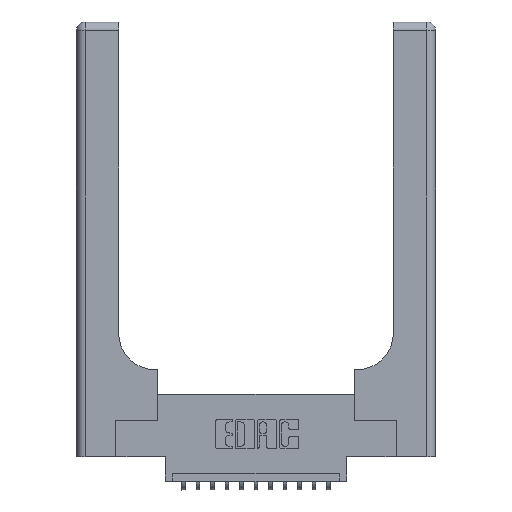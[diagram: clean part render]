
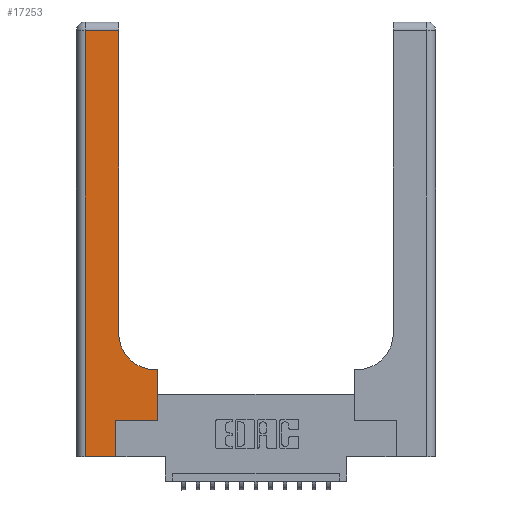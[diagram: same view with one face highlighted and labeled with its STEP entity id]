
A CAD part, top view. The second image highlights one B-rep face of the part: STEP entity #17253.
In plain terms, the highlighted planar face has unit normal (0, 0, 1).
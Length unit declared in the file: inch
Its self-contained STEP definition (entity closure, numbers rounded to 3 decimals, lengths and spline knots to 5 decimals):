
#71 = CARTESIAN_POINT ( 'NONE',  ( 0.269, 0.25, 0.37 ) ) ;
#83 = ORIENTED_EDGE ( 'NONE', *, *, #8795, .T. ) ;
#147 = AXIS2_PLACEMENT_3D ( 'NONE', #15369, #10408, #6244 ) ;
#502 = ORIENTED_EDGE ( 'NONE', *, *, #13716, .T. ) ;
#949 = EDGE_CURVE ( 'NONE', #11735, #5398, #17181, .T. ) ;
#1242 = CARTESIAN_POINT ( 'NONE',  ( 0.06, 3., 0.37 ) ) ;
#1856 = CARTESIAN_POINT ( 'NONE',  ( 0.06, 2.94, 0.37 ) ) ;
#2227 = DIRECTION ( 'NONE',  ( 0., 1., 0. ) ) ;
#2229 = CIRCLE ( 'NONE', #8083, 0.25 ) ;
#2405 = CARTESIAN_POINT ( 'NONE',  ( 0.269, 0., 0.37 ) ) ;
#2759 = VECTOR ( 'NONE', #15936, 39.37008 ) ;
#2775 = CARTESIAN_POINT ( 'NONE',  ( 0.06, 0., 0.37 ) ) ;
#2853 = CARTESIAN_POINT ( 'NONE',  ( 0.5585, 0.6, 0.37 ) ) ;
#2884 = VERTEX_POINT ( 'NONE', #9789 ) ;
#2964 = DIRECTION ( 'NONE',  ( 1., 0., 0. ) ) ;
#3438 = LINE ( 'NONE', #71, #13962 ) ;
#3503 = CARTESIAN_POINT ( 'NONE',  ( 0.2915, 3., 0.37 ) ) ;
#3720 = ORIENTED_EDGE ( 'NONE', *, *, #6353, .T. ) ;
#4133 = DIRECTION ( 'NONE',  ( 0., -1., 0. ) ) ;
#4957 = DIRECTION ( 'NONE',  ( -1., 0., 0. ) ) ;
#4966 = ORIENTED_EDGE ( 'NONE', *, *, #13176, .T. ) ;
#5148 = CARTESIAN_POINT ( 'NONE',  ( 0.5585, 0.25, 0.37 ) ) ;
#5274 = ORIENTED_EDGE ( 'NONE', *, *, #8549, .T. ) ;
#5398 = VERTEX_POINT ( 'NONE', #16535 ) ;
#5420 = VERTEX_POINT ( 'NONE', #6772 ) ;
#5808 = EDGE_LOOP ( 'NONE', ( #17011, #8208, #502, #4966, #7410, #14130, #3720, #83, #5274 ) ) ;
#6244 = DIRECTION ( 'NONE',  ( -1., 0., 0. ) ) ;
#6353 = EDGE_CURVE ( 'NONE', #7748, #11302, #6376, .T. ) ;
#6376 = LINE ( 'NONE', #5148, #11533 ) ;
#6515 = LINE ( 'NONE', #16203, #10816 ) ;
#6772 = CARTESIAN_POINT ( 'NONE',  ( 0.2915, 0.85, 0.37 ) ) ;
#7296 = VECTOR ( 'NONE', #2227, 39.37008 ) ;
#7410 = ORIENTED_EDGE ( 'NONE', *, *, #949, .T. ) ;
#7748 = VERTEX_POINT ( 'NONE', #16644 ) ;
#8083 = AXIS2_PLACEMENT_3D ( 'NONE', #11205, #10980, #2964 ) ;
#8169 = EDGE_CURVE ( 'NONE', #2884, #17229, #13679, .T. ) ;
#8208 = ORIENTED_EDGE ( 'NONE', *, *, #8169, .T. ) ;
#8503 = DIRECTION ( 'NONE',  ( 1., 0., 0. ) ) ;
#8549 = EDGE_CURVE ( 'NONE', #12171, #5420, #2229, .T. ) ;
#8795 = EDGE_CURVE ( 'NONE', #11302, #12171, #13235, .T. ) ;
#9048 = VERTEX_POINT ( 'NONE', #2775 ) ;
#9116 = CARTESIAN_POINT ( 'NONE',  ( 0.269, 0., 0.37 ) ) ;
#9351 = DIRECTION ( 'NONE',  ( -1., 0., 0. ) ) ;
#9527 = VECTOR ( 'NONE', #9351, 39.37008 ) ;
#9565 = VECTOR ( 'NONE', #4957, 39.37008 ) ;
#9789 = CARTESIAN_POINT ( 'NONE',  ( 0.2915, 2.94, 0.37 ) ) ;
#10408 = DIRECTION ( 'NONE',  ( 0., 0., -1. ) ) ;
#10785 = EDGE_CURVE ( 'NONE', #5420, #2884, #12293, .T. ) ;
#10816 = VECTOR ( 'NONE', #12349, 39.37008 ) ;
#10980 = DIRECTION ( 'NONE',  ( 0., 0., -1. ) ) ;
#11205 = CARTESIAN_POINT ( 'NONE',  ( 0.5415, 0.85, 0.37 ) ) ;
#11302 = VERTEX_POINT ( 'NONE', #2853 ) ;
#11391 = CARTESIAN_POINT ( 'NONE',  ( 0.5415, 0.6, 0.37 ) ) ;
#11533 = VECTOR ( 'NONE', #14836, 39.37008 ) ;
#11735 = VERTEX_POINT ( 'NONE', #9116 ) ;
#12171 = VERTEX_POINT ( 'NONE', #11391 ) ;
#12293 = LINE ( 'NONE', #3503, #7296 ) ;
#12315 = VECTOR ( 'NONE', #4133, 39.37008 ) ;
#12349 = DIRECTION ( 'NONE',  ( 1., 0., 0. ) ) ;
#12642 = PLANE ( 'NONE',  #147 ) ;
#13176 = EDGE_CURVE ( 'NONE', #9048, #11735, #6515, .T. ) ;
#13198 = LINE ( 'NONE', #1242, #12315 ) ;
#13232 = CARTESIAN_POINT ( 'NONE',  ( 0., 2.94, 0.37 ) ) ;
#13235 = LINE ( 'NONE', #16403, #9527 ) ;
#13679 = LINE ( 'NONE', #13232, #9565 ) ;
#13716 = EDGE_CURVE ( 'NONE', #17229, #9048, #13198, .T. ) ;
#13962 = VECTOR ( 'NONE', #8503, 39.37008 ) ;
#14130 = ORIENTED_EDGE ( 'NONE', *, *, #15879, .T. ) ;
#14563 = FACE_OUTER_BOUND ( 'NONE', #5808, .T. ) ;
#14836 = DIRECTION ( 'NONE',  ( 0., 1., 0. ) ) ;
#15369 = CARTESIAN_POINT ( 'NONE',  ( 0., 3., 0.37 ) ) ;
#15879 = EDGE_CURVE ( 'NONE', #5398, #7748, #3438, .T. ) ;
#15936 = DIRECTION ( 'NONE',  ( 0., 1., 0. ) ) ;
#16203 = CARTESIAN_POINT ( 'NONE',  ( 0., 0., 0.37 ) ) ;
#16403 = CARTESIAN_POINT ( 'NONE',  ( 0.2915, 0.6, 0.37 ) ) ;
#16535 = CARTESIAN_POINT ( 'NONE',  ( 0.269, 0.25, 0.37 ) ) ;
#16644 = CARTESIAN_POINT ( 'NONE',  ( 0.5585, 0.25, 0.37 ) ) ;
#17011 = ORIENTED_EDGE ( 'NONE', *, *, #10785, .T. ) ;
#17181 = LINE ( 'NONE', #2405, #2759 ) ;
#17229 = VERTEX_POINT ( 'NONE', #1856 ) ;
#17253 = ADVANCED_FACE ( 'NONE', ( #14563 ), #12642, .F. ) ;
